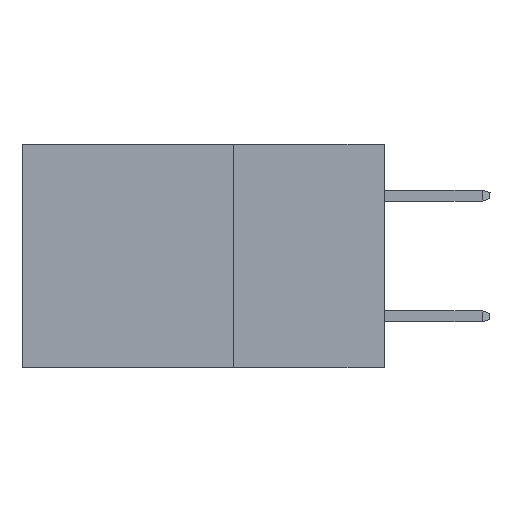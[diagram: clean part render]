
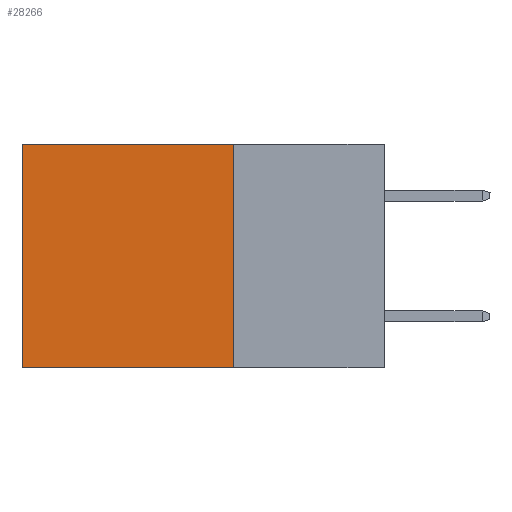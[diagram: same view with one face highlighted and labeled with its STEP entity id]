
A CAD part, left-side view. The second image highlights one B-rep face of the part: STEP entity #28266.
In plain terms, the highlighted planar face has unit normal (-1, 0, 0).
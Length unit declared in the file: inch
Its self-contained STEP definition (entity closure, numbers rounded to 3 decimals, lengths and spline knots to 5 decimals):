
#396 = EDGE_CURVE ( 'NONE', #29712, #10627, #25369, .T. ) ;
#2005 = VECTOR ( 'NONE', #27929, 39.37008 ) ;
#2527 = LINE ( 'NONE', #17744, #7379 ) ;
#5003 = CARTESIAN_POINT ( 'NONE',  ( 0.298, 0.25, 0. ) ) ;
#5569 = AXIS2_PLACEMENT_3D ( 'NONE', #27845, #13451, #30033 ) ;
#7379 = VECTOR ( 'NONE', #10851, 39.37008 ) ;
#7658 = CARTESIAN_POINT ( 'NONE',  ( 0.298, 0.25, 0. ) ) ;
#8339 = LINE ( 'NONE', #18842, #2005 ) ;
#10627 = VERTEX_POINT ( 'NONE', #18083 ) ;
#10851 = DIRECTION ( 'NONE',  ( 0., 0., -1. ) ) ;
#11860 = DIRECTION ( 'NONE',  ( 0., 0., -1. ) ) ;
#11980 = CARTESIAN_POINT ( 'NONE',  ( 0.298, 0.6, -0.37 ) ) ;
#12756 = VECTOR ( 'NONE', #28695, 39.37008 ) ;
#13451 = DIRECTION ( 'NONE',  ( 1., 0., 0. ) ) ;
#15034 = FACE_OUTER_BOUND ( 'NONE', #24192, .T. ) ;
#17340 = LINE ( 'NONE', #7658, #28511 ) ;
#17744 = CARTESIAN_POINT ( 'NONE',  ( 0.298, 0.6, 0. ) ) ;
#18083 = CARTESIAN_POINT ( 'NONE',  ( 0.298, 0.6, 0. ) ) ;
#18842 = CARTESIAN_POINT ( 'NONE',  ( 0.298, 0.25, -0.37 ) ) ;
#19659 = VERTEX_POINT ( 'NONE', #26464 ) ;
#20981 = ORIENTED_EDGE ( 'NONE', *, *, #26823, .F. ) ;
#24192 = EDGE_LOOP ( 'NONE', ( #28826, #26502, #20981, #26968 ) ) ;
#24538 = EDGE_CURVE ( 'NONE', #19659, #28938, #8339, .T. ) ;
#25369 = LINE ( 'NONE', #5003, #12756 ) ;
#25584 = PLANE ( 'NONE',  #5569 ) ;
#26464 = CARTESIAN_POINT ( 'NONE',  ( 0.298, 0.25, -0.37 ) ) ;
#26502 = ORIENTED_EDGE ( 'NONE', *, *, #24538, .F. ) ;
#26823 = EDGE_CURVE ( 'NONE', #29712, #19659, #17340, .T. ) ;
#26863 = CARTESIAN_POINT ( 'NONE',  ( 0.298, 0.25, 0. ) ) ;
#26968 = ORIENTED_EDGE ( 'NONE', *, *, #396, .T. ) ;
#27845 = CARTESIAN_POINT ( 'NONE',  ( 0.298, 0.25, 0. ) ) ;
#27893 = EDGE_CURVE ( 'NONE', #10627, #28938, #2527, .T. ) ;
#27929 = DIRECTION ( 'NONE',  ( 0., 1., 0. ) ) ;
#28266 = ADVANCED_FACE ( 'NONE', ( #15034 ), #25584, .F. ) ;
#28511 = VECTOR ( 'NONE', #11860, 39.37008 ) ;
#28695 = DIRECTION ( 'NONE',  ( 0., 1., 0. ) ) ;
#28826 = ORIENTED_EDGE ( 'NONE', *, *, #27893, .T. ) ;
#28938 = VERTEX_POINT ( 'NONE', #11980 ) ;
#29712 = VERTEX_POINT ( 'NONE', #26863 ) ;
#30033 = DIRECTION ( 'NONE',  ( 0., 0., -1. ) ) ;
